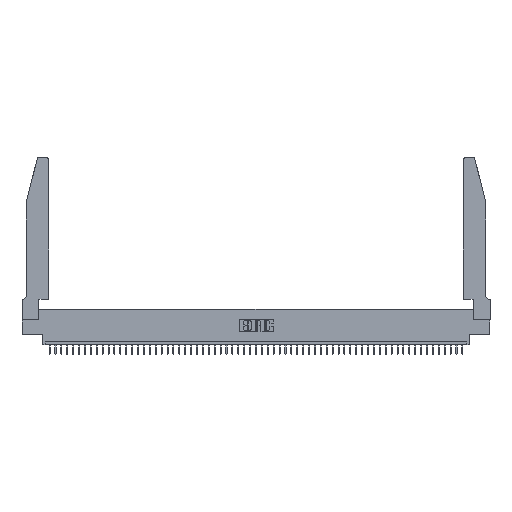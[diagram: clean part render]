
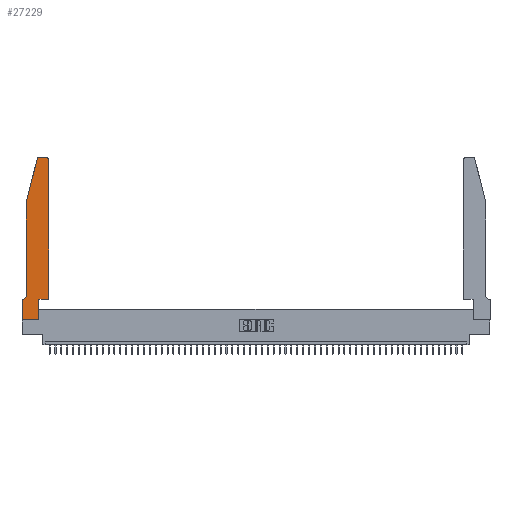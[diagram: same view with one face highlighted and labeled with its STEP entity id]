
A CAD part, top view. The second image highlights one B-rep face of the part: STEP entity #27229.
In plain terms, the highlighted planar face has unit normal (0, 0, 1).
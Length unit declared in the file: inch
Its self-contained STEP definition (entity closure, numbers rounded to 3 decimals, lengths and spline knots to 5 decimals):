
#656 = DIRECTION ( 'NONE',  ( 0., 0., 1. ) ) ;
#862 = AXIS2_PLACEMENT_3D ( 'NONE', #2229, #48763, #52788 ) ;
#1089 = VERTEX_POINT ( 'NONE', #37992 ) ;
#1247 = CARTESIAN_POINT ( 'NONE',  ( 0.0755, 2., 0.37 ) ) ;
#1733 = DIRECTION ( 'NONE',  ( 1., 0., 0. ) ) ;
#1867 = CARTESIAN_POINT ( 'NONE',  ( 0.4205, 2.75, 0.37 ) ) ;
#2229 = CARTESIAN_POINT ( 'NONE',  ( 0.284, 2.72, 0.37 ) ) ;
#3823 = VECTOR ( 'NONE', #51521, 39.37008 ) ;
#4168 = VERTEX_POINT ( 'NONE', #7422 ) ;
#5487 = CARTESIAN_POINT ( 'NONE',  ( 0.0755, 2., 0.37 ) ) ;
#5736 = VECTOR ( 'NONE', #47972, 39.37008 ) ;
#6199 = LINE ( 'NONE', #5487, #49665 ) ;
#6403 = LINE ( 'NONE', #34568, #3823 ) ;
#6417 = VERTEX_POINT ( 'NONE', #29104 ) ;
#6720 = DIRECTION ( 'NONE',  ( 0., 0., 1. ) ) ;
#7422 = CARTESIAN_POINT ( 'NONE',  ( 0.25487, 2.72718, 0.37 ) ) ;
#7423 = EDGE_CURVE ( 'NONE', #38439, #52316, #6199, .T. ) ;
#7541 = DIRECTION ( 'NONE',  ( -1., 0., 0. ) ) ;
#8442 = DIRECTION ( 'NONE',  ( 1., 0., 0. ) ) ;
#9982 = VERTEX_POINT ( 'NONE', #37307 ) ;
#10387 = VERTEX_POINT ( 'NONE', #1867 ) ;
#11377 = ORIENTED_EDGE ( 'NONE', *, *, #43807, .T. ) ;
#11429 = ORIENTED_EDGE ( 'NONE', *, *, #35181, .T. ) ;
#11677 = EDGE_CURVE ( 'NONE', #9982, #53886, #18334, .T. ) ;
#14602 = CIRCLE ( 'NONE', #51065, 0.03 ) ;
#14996 = AXIS2_PLACEMENT_3D ( 'NONE', #42104, #656, #8442 ) ;
#15091 = VECTOR ( 'NONE', #42545, 39.37008 ) ;
#16387 = EDGE_CURVE ( 'NONE', #25334, #21133, #6403, .T. ) ;
#16827 = DIRECTION ( 'NONE',  ( 0., 0., -1. ) ) ;
#16937 = LINE ( 'NONE', #17110, #31368 ) ;
#17110 = CARTESIAN_POINT ( 'NONE',  ( 0.0755, 0.35, 0.37 ) ) ;
#17670 = CARTESIAN_POINT ( 'NONE',  ( 0.2865, 0.35, 0.37 ) ) ;
#17814 = FACE_OUTER_BOUND ( 'NONE', #53605, .T. ) ;
#18196 = CARTESIAN_POINT ( 'NONE',  ( 0.2605, 2.75, 0.37 ) ) ;
#18334 = LINE ( 'NONE', #49388, #26867 ) ;
#19420 = DIRECTION ( 'NONE',  ( 0., 1., 0. ) ) ;
#20297 = CARTESIAN_POINT ( 'NONE',  ( 0., 0., 0.37 ) ) ;
#21059 = DIRECTION ( 'NONE',  ( -1., 0., 0. ) ) ;
#21133 = VERTEX_POINT ( 'NONE', #20297 ) ;
#21753 = CARTESIAN_POINT ( 'NONE',  ( 0.0055, 0.42, 0.37 ) ) ;
#21816 = ORIENTED_EDGE ( 'NONE', *, *, #7423, .T. ) ;
#22445 = ORIENTED_EDGE ( 'NONE', *, *, #27935, .T. ) ;
#23011 = CIRCLE ( 'NONE', #862, 0.03 ) ;
#23049 = LINE ( 'NONE', #33224, #40105 ) ;
#25259 = ORIENTED_EDGE ( 'NONE', *, *, #39288, .T. ) ;
#25334 = VERTEX_POINT ( 'NONE', #27169 ) ;
#26642 = DIRECTION ( 'NONE',  ( -1., 0., 0. ) ) ;
#26867 = VECTOR ( 'NONE', #19420, 39.37008 ) ;
#27169 = CARTESIAN_POINT ( 'NONE',  ( 0., 0.35, 0.37 ) ) ;
#27229 = ADVANCED_FACE ( 'NONE', ( #17814 ), #46846, .T. ) ;
#27555 = ORIENTED_EDGE ( 'NONE', *, *, #43285, .T. ) ;
#27866 = ORIENTED_EDGE ( 'NONE', *, *, #11677, .T. ) ;
#27935 = EDGE_CURVE ( 'NONE', #4168, #38439, #23049, .T. ) ;
#29104 = CARTESIAN_POINT ( 'NONE',  ( 0.2865, 0.35, 0.37 ) ) ;
#30343 = EDGE_CURVE ( 'NONE', #52006, #25334, #16937, .T. ) ;
#31368 = VECTOR ( 'NONE', #7541, 39.37008 ) ;
#32321 = CARTESIAN_POINT ( 'NONE',  ( 0.0755, 0.42, 0.37 ) ) ;
#33224 = CARTESIAN_POINT ( 'NONE',  ( 0.0755, 2., 0.37 ) ) ;
#33499 = CARTESIAN_POINT ( 'NONE',  ( 0.4505, 2.72, 0.37 ) ) ;
#34066 = VERTEX_POINT ( 'NONE', #43103 ) ;
#34568 = CARTESIAN_POINT ( 'NONE',  ( 0., 0., 0.37 ) ) ;
#35120 = ORIENTED_EDGE ( 'NONE', *, *, #16387, .T. ) ;
#35181 = EDGE_CURVE ( 'NONE', #21133, #34066, #47847, .T. ) ;
#35518 = LINE ( 'NONE', #17670, #43459 ) ;
#35598 = CARTESIAN_POINT ( 'NONE',  ( 0., 0., 0.37 ) ) ;
#35669 = ORIENTED_EDGE ( 'NONE', *, *, #48033, .T. ) ;
#37307 = CARTESIAN_POINT ( 'NONE',  ( 0.4505, 0.35, 0.37 ) ) ;
#37992 = CARTESIAN_POINT ( 'NONE',  ( 0.284, 2.75, 0.37 ) ) ;
#38439 = VERTEX_POINT ( 'NONE', #1247 ) ;
#39234 = CARTESIAN_POINT ( 'NONE',  ( 0.0055, 0.35, 0.37 ) ) ;
#39288 = EDGE_CURVE ( 'NONE', #1089, #4168, #23011, .T. ) ;
#40048 = LINE ( 'NONE', #46586, #15091 ) ;
#40105 = VECTOR ( 'NONE', #41514, 39.37008 ) ;
#41514 = DIRECTION ( 'NONE',  ( -0.239, -0.971, 0. ) ) ;
#42104 = CARTESIAN_POINT ( 'NONE',  ( 0., 0.35, 0.37 ) ) ;
#42363 = AXIS2_PLACEMENT_3D ( 'NONE', #21753, #16827, #21059 ) ;
#42545 = DIRECTION ( 'NONE',  ( 1., 0., 0. ) ) ;
#42938 = ORIENTED_EDGE ( 'NONE', *, *, #48028, .T. ) ;
#43103 = CARTESIAN_POINT ( 'NONE',  ( 0.2865, 0., 0.37 ) ) ;
#43285 = EDGE_CURVE ( 'NONE', #53886, #10387, #14602, .T. ) ;
#43459 = VECTOR ( 'NONE', #47488, 39.37008 ) ;
#43807 = EDGE_CURVE ( 'NONE', #34066, #6417, #35518, .T. ) ;
#45539 = ORIENTED_EDGE ( 'NONE', *, *, #30343, .T. ) ;
#46586 = CARTESIAN_POINT ( 'NONE',  ( 0.4505, 0.35, 0.37 ) ) ;
#46846 = PLANE ( 'NONE',  #14996 ) ;
#47488 = DIRECTION ( 'NONE',  ( 0., 1., 0. ) ) ;
#47847 = LINE ( 'NONE', #35598, #5736 ) ;
#47972 = DIRECTION ( 'NONE',  ( 1., 0., 0. ) ) ;
#48028 = EDGE_CURVE ( 'NONE', #6417, #9982, #40048, .T. ) ;
#48033 = EDGE_CURVE ( 'NONE', #52316, #52006, #50653, .T. ) ;
#48648 = CARTESIAN_POINT ( 'NONE',  ( 0.4205, 2.72, 0.37 ) ) ;
#48763 = DIRECTION ( 'NONE',  ( 0., 0., 1. ) ) ;
#49388 = CARTESIAN_POINT ( 'NONE',  ( 0.4505, 0.35, 0.37 ) ) ;
#49665 = VECTOR ( 'NONE', #51773, 39.37008 ) ;
#50611 = LINE ( 'NONE', #18196, #53244 ) ;
#50653 = CIRCLE ( 'NONE', #42363, 0.07 ) ;
#50857 = ORIENTED_EDGE ( 'NONE', *, *, #51343, .T. ) ;
#51065 = AXIS2_PLACEMENT_3D ( 'NONE', #48648, #6720, #1733 ) ;
#51343 = EDGE_CURVE ( 'NONE', #10387, #1089, #50611, .T. ) ;
#51521 = DIRECTION ( 'NONE',  ( 0., -1., 0. ) ) ;
#51773 = DIRECTION ( 'NONE',  ( 0., -1., 0. ) ) ;
#52006 = VERTEX_POINT ( 'NONE', #39234 ) ;
#52316 = VERTEX_POINT ( 'NONE', #32321 ) ;
#52788 = DIRECTION ( 'NONE',  ( 1., 0., 0. ) ) ;
#53244 = VECTOR ( 'NONE', #26642, 39.37008 ) ;
#53605 = EDGE_LOOP ( 'NONE', ( #50857, #25259, #22445, #21816, #35669, #45539, #35120, #11429, #11377, #42938, #27866, #27555 ) ) ;
#53886 = VERTEX_POINT ( 'NONE', #33499 ) ;
